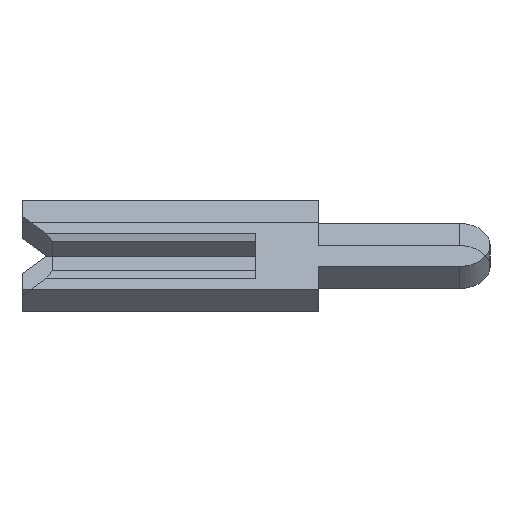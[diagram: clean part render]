
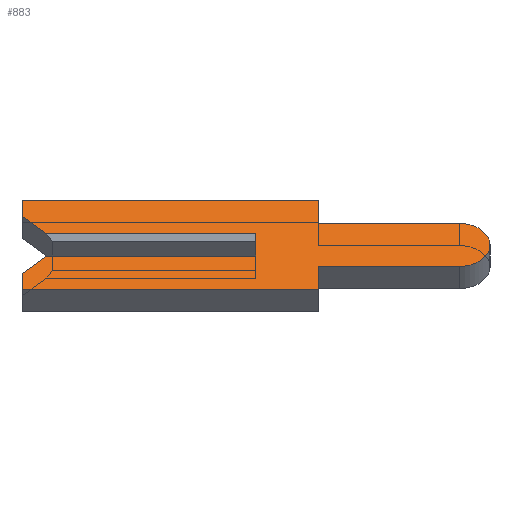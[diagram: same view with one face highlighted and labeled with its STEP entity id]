
A CAD part, left-side view. The second image highlights one B-rep face of the part: STEP entity #883.
In plain terms, the highlighted face is planar.
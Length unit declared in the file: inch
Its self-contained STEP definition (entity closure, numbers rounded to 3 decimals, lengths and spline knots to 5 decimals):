
#25 = ORIENTED_EDGE ( 'NONE', *, *, #1019, .F. ) ;
#42 = VECTOR ( 'NONE', #1605, 39.37008 ) ;
#70 = CARTESIAN_POINT ( 'NONE',  ( -0.01, -0.04, 0.0195 ) ) ;
#97 = CARTESIAN_POINT ( 'NONE',  ( -0.01, -0.04, 0.0195 ) ) ;
#118 = VECTOR ( 'NONE', #2066, 39.37008 ) ;
#148 = CARTESIAN_POINT ( 'NONE',  ( -0.01, 0., 0.01 ) ) ;
#169 = VECTOR ( 'NONE', #1842, 39.37008 ) ;
#225 = VERTEX_POINT ( 'NONE', #777 ) ;
#239 = ORIENTED_EDGE ( 'NONE', *, *, #358, .T. ) ;
#271 = EDGE_CURVE ( 'NONE', #1831, #711, #716, .T. ) ;
#280 = EDGE_CURVE ( 'NONE', #225, #1228, #924, .T. ) ;
#319 = EDGE_CURVE ( 'NONE', #668, #996, #1446, .T. ) ;
#333 = VECTOR ( 'NONE', #1359, 39.37008 ) ;
#340 = CARTESIAN_POINT ( 'NONE',  ( -0.01, 0.15, 0.04 ) ) ;
#344 = CARTESIAN_POINT ( 'NONE',  ( -0.01, 0.15, -0.026 ) ) ;
#350 = CARTESIAN_POINT ( 'NONE',  ( -0.01, 0.15, 0.026 ) ) ;
#358 = EDGE_CURVE ( 'NONE', #1901, #571, #480, .T. ) ;
#370 = CARTESIAN_POINT ( 'NONE',  ( -0.01, -0.1305, 0. ) ) ;
#379 = VECTOR ( 'NONE', #2071, 39.37008 ) ;
#419 = ORIENTED_EDGE ( 'NONE', *, *, #1141, .F. ) ;
#440 = CARTESIAN_POINT ( 'NONE',  ( -0.01, -0.1305, -0.01 ) ) ;
#480 = LINE ( 'NONE', #640, #1404 ) ;
#491 = CARTESIAN_POINT ( 'NONE',  ( -0.01, -0.1305, 0. ) ) ;
#504 = ORIENTED_EDGE ( 'NONE', *, *, #2015, .F. ) ;
#511 = CARTESIAN_POINT ( 'NONE',  ( -0.01, 0., -0.01 ) ) ;
#515 = DIRECTION ( 'NONE',  ( 0., 0., 1. ) ) ;
#569 = CARTESIAN_POINT ( 'NONE',  ( -0.01, 0., 0.0065 ) ) ;
#571 = VERTEX_POINT ( 'NONE', #148 ) ;
#578 = LINE ( 'NONE', #350, #333 ) ;
#595 = EDGE_CURVE ( 'NONE', #799, #1831, #1325, .T. ) ;
#630 = DIRECTION ( 'NONE',  ( 0., -1., 0. ) ) ;
#633 = LINE ( 'NONE', #569, #1185 ) ;
#640 = CARTESIAN_POINT ( 'NONE',  ( -0.01, 0.15, 0.01 ) ) ;
#668 = VERTEX_POINT ( 'NONE', #964 ) ;
#711 = VERTEX_POINT ( 'NONE', #511 ) ;
#716 = LINE ( 'NONE', #440, #118 ) ;
#721 = EDGE_CURVE ( 'NONE', #1228, #799, #1905, .T. ) ;
#722 = ORIENTED_EDGE ( 'NONE', *, *, #595, .F. ) ;
#751 = CARTESIAN_POINT ( 'NONE',  ( -0.01, -0.04, -0.0195 ) ) ;
#774 = ORIENTED_EDGE ( 'NONE', *, *, #1840, .F. ) ;
#777 = CARTESIAN_POINT ( 'NONE',  ( -0.01, -0.04, -0.04 ) ) ;
#789 = EDGE_CURVE ( 'NONE', #1090, #1810, #1353, .T. ) ;
#799 = VERTEX_POINT ( 'NONE', #1658 ) ;
#815 = LINE ( 'NONE', #1430, #379 ) ;
#819 = VECTOR ( 'NONE', #1631, 39.37008 ) ;
#838 = CARTESIAN_POINT ( 'NONE',  ( -0.01, 0.15, 0.04 ) ) ;
#869 = VECTOR ( 'NONE', #1615, 39.37008 ) ;
#879 = DIRECTION ( 'NONE',  ( 0., 0., -1. ) ) ;
#881 = ORIENTED_EDGE ( 'NONE', *, *, #1306, .F. ) ;
#883 = ADVANCED_FACE ( 'NONE', ( #1297 ), #1010, .F. ) ;
#890 = DIRECTION ( 'NONE',  ( 0., 0.707, 0.707 ) ) ;
#902 = CARTESIAN_POINT ( 'NONE',  ( -0.01, 0.134, 0.01 ) ) ;
#908 = DIRECTION ( 'NONE',  ( 0., 0., 1. ) ) ;
#922 = ORIENTED_EDGE ( 'NONE', *, *, #721, .F. ) ;
#924 = LINE ( 'NONE', #1934, #819 ) ;
#927 = CARTESIAN_POINT ( 'NONE',  ( -0.01, -0.1305, 0.0195 ) ) ;
#964 = CARTESIAN_POINT ( 'NONE',  ( -0.01, -0.1305, -0.0195 ) ) ;
#996 = VERTEX_POINT ( 'NONE', #1514 ) ;
#1010 = PLANE ( 'NONE',  #1265 ) ;
#1019 = EDGE_CURVE ( 'NONE', #1591, #1090, #578, .T. ) ;
#1028 = ORIENTED_EDGE ( 'NONE', *, *, #789, .F. ) ;
#1088 = ORIENTED_EDGE ( 'NONE', *, *, #280, .F. ) ;
#1090 = VERTEX_POINT ( 'NONE', #838 ) ;
#1141 = EDGE_CURVE ( 'NONE', #1883, #1508, #2031, .T. ) ;
#1154 = VECTOR ( 'NONE', #879, 39.37008 ) ;
#1185 = VECTOR ( 'NONE', #908, 39.37008 ) ;
#1228 = VERTEX_POINT ( 'NONE', #1553 ) ;
#1255 = CARTESIAN_POINT ( 'NONE',  ( -0.01, 0.15, 0.026 ) ) ;
#1265 = AXIS2_PLACEMENT_3D ( 'NONE', #491, #1987, #1663 ) ;
#1290 = CARTESIAN_POINT ( 'NONE',  ( -0.01, 0.1305, -0.0065 ) ) ;
#1297 = FACE_OUTER_BOUND ( 'NONE', #1361, .T. ) ;
#1306 = EDGE_CURVE ( 'NONE', #1508, #668, #2076, .T. ) ;
#1325 = LINE ( 'NONE', #1290, #869 ) ;
#1353 = LINE ( 'NONE', #340, #169 ) ;
#1359 = DIRECTION ( 'NONE',  ( 0., 0., 1. ) ) ;
#1361 = EDGE_LOOP ( 'NONE', ( #239, #774, #1676, #722, #922, #1088, #504, #1593, #881, #419, #1991, #1028, #25, #2034 ) ) ;
#1364 = DIRECTION ( 'NONE',  ( 1., 0., 0. ) ) ;
#1404 = VECTOR ( 'NONE', #630, 39.37008 ) ;
#1414 = CARTESIAN_POINT ( 'NONE',  ( -0.01, 0.1305, 0.0065 ) ) ;
#1430 = CARTESIAN_POINT ( 'NONE',  ( -0.01, -0.04, -0.04 ) ) ;
#1446 = LINE ( 'NONE', #751, #42 ) ;
#1477 = VECTOR ( 'NONE', #890, 39.37008 ) ;
#1479 = VECTOR ( 'NONE', #515, 39.37008 ) ;
#1488 = EDGE_CURVE ( 'NONE', #1810, #1883, #1703, .T. ) ;
#1508 = VERTEX_POINT ( 'NONE', #927 ) ;
#1514 = CARTESIAN_POINT ( 'NONE',  ( -0.01, -0.04, -0.0195 ) ) ;
#1537 = DIRECTION ( 'NONE',  ( 0., 0., -1. ) ) ;
#1553 = CARTESIAN_POINT ( 'NONE',  ( -0.01, 0.15, -0.04 ) ) ;
#1570 = CARTESIAN_POINT ( 'NONE',  ( -0.01, -0.04, 0.04 ) ) ;
#1591 = VERTEX_POINT ( 'NONE', #1255 ) ;
#1593 = ORIENTED_EDGE ( 'NONE', *, *, #319, .F. ) ;
#1605 = DIRECTION ( 'NONE',  ( 0., 1., 0. ) ) ;
#1615 = DIRECTION ( 'NONE',  ( 0., -0.707, 0.707 ) ) ;
#1631 = DIRECTION ( 'NONE',  ( 0., 1., 0. ) ) ;
#1658 = CARTESIAN_POINT ( 'NONE',  ( -0.01, 0.15, -0.026 ) ) ;
#1663 = DIRECTION ( 'NONE',  ( 0., 0., -1. ) ) ;
#1676 = ORIENTED_EDGE ( 'NONE', *, *, #271, .F. ) ;
#1684 = EDGE_CURVE ( 'NONE', #1901, #1591, #2058, .T. ) ;
#1703 = LINE ( 'NONE', #2036, #1154 ) ;
#1712 = DIRECTION ( 'NONE',  ( 0., -1., 0. ) ) ;
#1731 = VECTOR ( 'NONE', #1712, 39.37008 ) ;
#1810 = VERTEX_POINT ( 'NONE', #1570 ) ;
#1831 = VERTEX_POINT ( 'NONE', #1882 ) ;
#1840 = EDGE_CURVE ( 'NONE', #711, #571, #633, .T. ) ;
#1842 = DIRECTION ( 'NONE',  ( 0., -1., 0. ) ) ;
#1882 = CARTESIAN_POINT ( 'NONE',  ( -0.01, 0.134, -0.01 ) ) ;
#1883 = VERTEX_POINT ( 'NONE', #97 ) ;
#1887 = AXIS2_PLACEMENT_3D ( 'NONE', #370, #1364, #1537 ) ;
#1901 = VERTEX_POINT ( 'NONE', #902 ) ;
#1905 = LINE ( 'NONE', #344, #1479 ) ;
#1934 = CARTESIAN_POINT ( 'NONE',  ( -0.01, 0.15, -0.04 ) ) ;
#1987 = DIRECTION ( 'NONE',  ( 1., 0., 0. ) ) ;
#1991 = ORIENTED_EDGE ( 'NONE', *, *, #1488, .F. ) ;
#2015 = EDGE_CURVE ( 'NONE', #996, #225, #815, .T. ) ;
#2031 = LINE ( 'NONE', #70, #1731 ) ;
#2034 = ORIENTED_EDGE ( 'NONE', *, *, #1684, .F. ) ;
#2036 = CARTESIAN_POINT ( 'NONE',  ( -0.01, -0.04, 0.04 ) ) ;
#2058 = LINE ( 'NONE', #1414, #1477 ) ;
#2066 = DIRECTION ( 'NONE',  ( 0., -1., 0. ) ) ;
#2071 = DIRECTION ( 'NONE',  ( 0., 0., -1. ) ) ;
#2076 = CIRCLE ( 'NONE', #1887, 0.0195 ) ;
